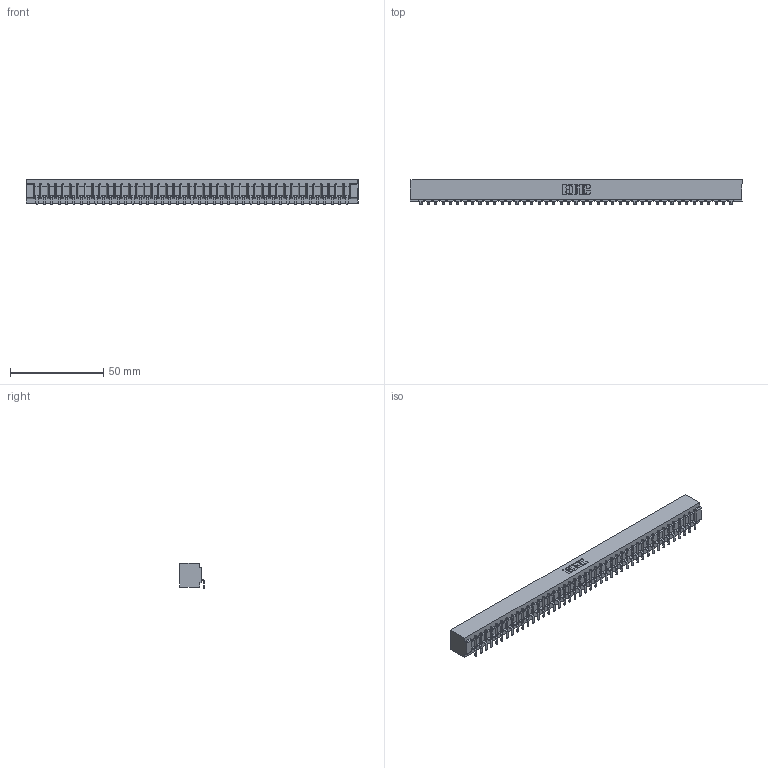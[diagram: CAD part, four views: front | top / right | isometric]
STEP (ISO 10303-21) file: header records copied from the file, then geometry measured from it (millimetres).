
FILE_DESCRIPTION (( 'STEP AP203' ), '1' );
FILE_NAME ('357-043-553-101.STEP', '2019-09-17T11:05:50', ( '' ), ( '' ), 'SwSTEP 2.0', 'SolidWorks 2016', '' );
FILE_SCHEMA (( 'CONFIG_CONTROL_DESIGN' ));
Length unit declared in the file: inch
Products named in the file (3): 307 Part_No Mounting Lugs; 307-290-002_553; 357-043-553-101
Assembly tree (44 placements, depth 2):
  357-043-553-101
    307 Part_No Mounting Lugs
    307-290-002_553  x43
Bounding box: 178.26 x 13.32 x 13.5 mm (x, y, z)
Volume: 19640.8 mm3; surface area: 25059.8 mm2
Topology: 44 solids, 44 shells, 3508 faces, 10791 edges, 7074 vertices
Faces by surface type: plane 2087, cylinder 1333, sphere 88
Entity records: 37316 total; most frequent: CARTESIAN_POINT 6296, ORIENTED_EDGE 6286, DIRECTION 6115, EDGE_CURVE 3143, VECTOR 2409, LINE 2409, VERTEX_POINT 2034, AXIS2_PLACEMENT_3D 1853
